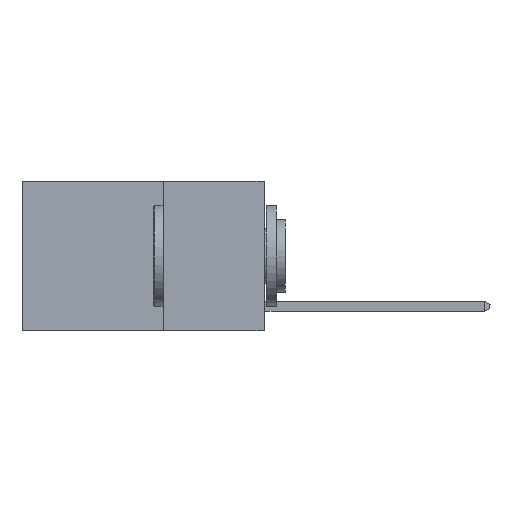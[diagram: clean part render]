
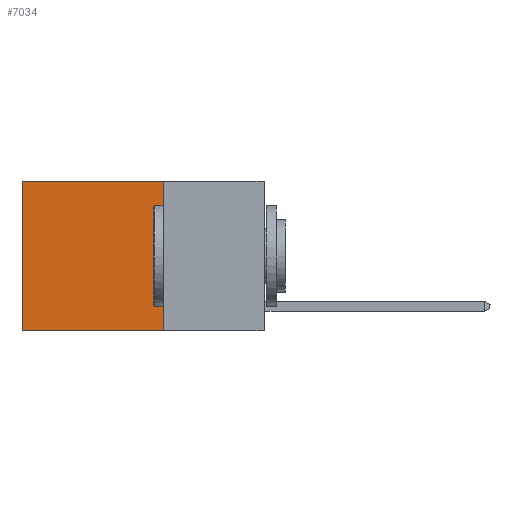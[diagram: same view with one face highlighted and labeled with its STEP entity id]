
A CAD part, left-side view. The second image highlights one B-rep face of the part: STEP entity #7034.
In plain terms, the highlighted planar face has unit normal (-1, 0, 0).
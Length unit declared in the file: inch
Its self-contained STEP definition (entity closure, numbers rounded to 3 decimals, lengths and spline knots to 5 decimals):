
#333 = CARTESIAN_POINT ( 'NONE',  ( 0.2625, 0.6, -0.37 ) ) ;
#342 = DIRECTION ( 'NONE',  ( 0., 0., -1. ) ) ;
#525 = CARTESIAN_POINT ( 'NONE',  ( 0.2625, 0.6, 0. ) ) ;
#2033 = VECTOR ( 'NONE', #11106, 39.37008 ) ;
#2543 = VERTEX_POINT ( 'NONE', #525 ) ;
#2731 = VECTOR ( 'NONE', #7667, 39.37008 ) ;
#2876 = CARTESIAN_POINT ( 'NONE',  ( 0.2625, 0.25, 0. ) ) ;
#3199 = PLANE ( 'NONE',  #9234 ) ;
#3329 = VERTEX_POINT ( 'NONE', #5148 ) ;
#4002 = DIRECTION ( 'NONE',  ( 1., 0., 0. ) ) ;
#4036 = DIRECTION ( 'NONE',  ( 0., 0., -1. ) ) ;
#4135 = CARTESIAN_POINT ( 'NONE',  ( 0.2625, 0.25, 0. ) ) ;
#4398 = EDGE_CURVE ( 'NONE', #3329, #11051, #7227, .T. ) ;
#4638 = EDGE_CURVE ( 'NONE', #4737, #3329, #9689, .T. ) ;
#4669 = CARTESIAN_POINT ( 'NONE',  ( 0.2625, 0.25, -0.37 ) ) ;
#4737 = VERTEX_POINT ( 'NONE', #4135 ) ;
#4955 = LINE ( 'NONE', #5073, #2731 ) ;
#5073 = CARTESIAN_POINT ( 'NONE',  ( 0.2625, 0.6, 0. ) ) ;
#5148 = CARTESIAN_POINT ( 'NONE',  ( 0.2625, 0.25, -0.37 ) ) ;
#5228 = EDGE_LOOP ( 'NONE', ( #10609, #10638, #10715, #10757 ) ) ;
#5297 = VECTOR ( 'NONE', #342, 39.37008 ) ;
#5446 = VECTOR ( 'NONE', #9622, 39.37008 ) ;
#6565 = LINE ( 'NONE', #2876, #2033 ) ;
#7034 = ADVANCED_FACE ( 'NONE', ( #8047 ), #3199, .F. ) ;
#7227 = LINE ( 'NONE', #4669, #5446 ) ;
#7448 = CARTESIAN_POINT ( 'NONE',  ( 0.2625, 0.25, 0. ) ) ;
#7667 = DIRECTION ( 'NONE',  ( 0., 0., -1. ) ) ;
#8047 = FACE_OUTER_BOUND ( 'NONE', #5228, .T. ) ;
#9234 = AXIS2_PLACEMENT_3D ( 'NONE', #7448, #4002, #4036 ) ;
#9622 = DIRECTION ( 'NONE',  ( 0., 1., 0. ) ) ;
#9689 = LINE ( 'NONE', #9831, #5297 ) ;
#9831 = CARTESIAN_POINT ( 'NONE',  ( 0.2625, 0.25, 0. ) ) ;
#10059 = EDGE_CURVE ( 'NONE', #2543, #11051, #4955, .T. ) ;
#10609 = ORIENTED_EDGE ( 'NONE', *, *, #10059, .T. ) ;
#10638 = ORIENTED_EDGE ( 'NONE', *, *, #4398, .F. ) ;
#10715 = ORIENTED_EDGE ( 'NONE', *, *, #4638, .F. ) ;
#10757 = ORIENTED_EDGE ( 'NONE', *, *, #10861, .T. ) ;
#10861 = EDGE_CURVE ( 'NONE', #4737, #2543, #6565, .T. ) ;
#11051 = VERTEX_POINT ( 'NONE', #333 ) ;
#11106 = DIRECTION ( 'NONE',  ( 0., 1., 0. ) ) ;
